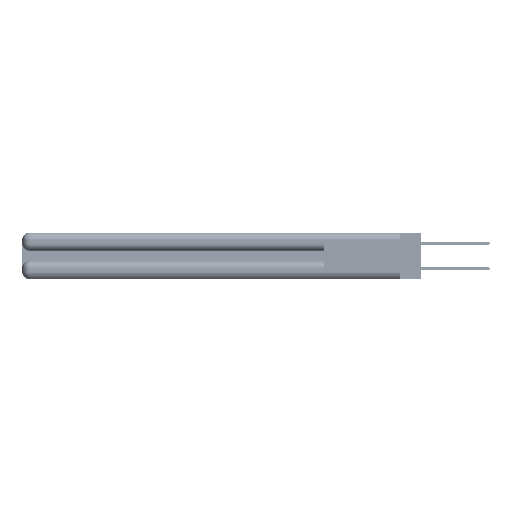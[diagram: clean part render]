
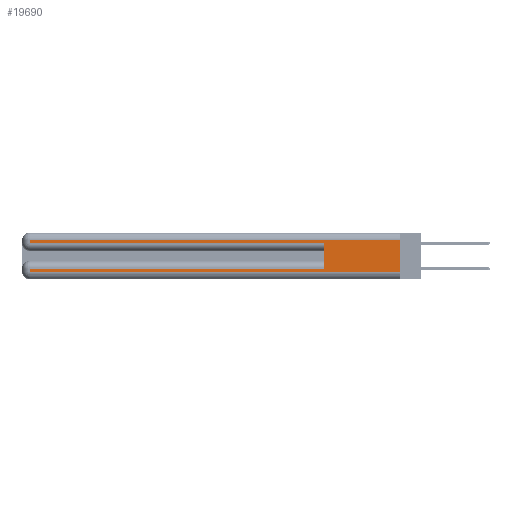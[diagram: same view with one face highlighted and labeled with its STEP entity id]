
A CAD part, left-side view. The second image highlights one B-rep face of the part: STEP entity #19690.
In plain terms, the highlighted planar face has unit normal (-1, 0, 0).
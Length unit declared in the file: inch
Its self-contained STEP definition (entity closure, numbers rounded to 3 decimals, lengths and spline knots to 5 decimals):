
#642 = EDGE_CURVE ( 'NONE', #25531, #5206, #15924, .T. ) ;
#791 = DIRECTION ( 'NONE',  ( 0., 0., -1. ) ) ;
#2185 = LINE ( 'NONE', #38076, #24866 ) ;
#4907 = PLANE ( 'NONE',  #18648 ) ;
#5204 = ORIENTED_EDGE ( 'NONE', *, *, #642, .F. ) ;
#5206 = VERTEX_POINT ( 'NONE', #48222 ) ;
#6239 = VECTOR ( 'NONE', #22172, 39.37008 ) ;
#6719 = VECTOR ( 'NONE', #21812, 39.37008 ) ;
#8620 = CARTESIAN_POINT ( 'NONE',  ( 0., 0., 0.31 ) ) ;
#8904 = EDGE_LOOP ( 'NONE', ( #52292, #32001, #41265, #22554, #5204, #45178, #51805, #26431 ) ) ;
#9344 = LINE ( 'NONE', #25395, #31962 ) ;
#10010 = EDGE_CURVE ( 'NONE', #43387, #15012, #35726, .T. ) ;
#10429 = VECTOR ( 'NONE', #53591, 39.37008 ) ;
#13871 = DIRECTION ( 'NONE',  ( 0., 1., 0. ) ) ;
#14803 = VERTEX_POINT ( 'NONE', #8620 ) ;
#15012 = VERTEX_POINT ( 'NONE', #43968 ) ;
#15924 = LINE ( 'NONE', #39296, #37211 ) ;
#16337 = CARTESIAN_POINT ( 'NONE',  ( 0., 2.94, 0.285 ) ) ;
#17550 = CARTESIAN_POINT ( 'NONE',  ( 0., 2.94, 0.37 ) ) ;
#17668 = EDGE_CURVE ( 'NONE', #43032, #5206, #2185, .T. ) ;
#17908 = CARTESIAN_POINT ( 'NONE',  ( 0., 0., 0.37 ) ) ;
#18648 = AXIS2_PLACEMENT_3D ( 'NONE', #43265, #26305, #791 ) ;
#19479 = CARTESIAN_POINT ( 'NONE',  ( 0., 0., 0.06 ) ) ;
#19516 = EDGE_CURVE ( 'NONE', #14803, #42316, #9344, .T. ) ;
#19690 = ADVANCED_FACE ( 'NONE', ( #33978 ), #4907, .F. ) ;
#21027 = CARTESIAN_POINT ( 'NONE',  ( 0., 2.94, 0.085 ) ) ;
#21812 = DIRECTION ( 'NONE',  ( 0., 0., -1. ) ) ;
#21819 = EDGE_CURVE ( 'NONE', #42316, #43032, #52481, .T. ) ;
#22172 = DIRECTION ( 'NONE',  ( 0., 0., -1. ) ) ;
#22333 = DIRECTION ( 'NONE',  ( 0., 0., 1. ) ) ;
#22554 = ORIENTED_EDGE ( 'NONE', *, *, #17668, .T. ) ;
#23905 = CARTESIAN_POINT ( 'NONE',  ( 0., 0.6, 0.085 ) ) ;
#24866 = VECTOR ( 'NONE', #42327, 39.37008 ) ;
#25395 = CARTESIAN_POINT ( 'NONE',  ( 0., 0., 0.31 ) ) ;
#25531 = VERTEX_POINT ( 'NONE', #23905 ) ;
#26305 = DIRECTION ( 'NONE',  ( 1., 0., 0. ) ) ;
#26395 = VERTEX_POINT ( 'NONE', #21027 ) ;
#26431 = ORIENTED_EDGE ( 'NONE', *, *, #10010, .T. ) ;
#26536 = EDGE_CURVE ( 'NONE', #14803, #15012, #51573, .T. ) ;
#28405 = EDGE_CURVE ( 'NONE', #26395, #43387, #40731, .T. ) ;
#29588 = VECTOR ( 'NONE', #13871, 39.37008 ) ;
#31962 = VECTOR ( 'NONE', #50518, 39.37008 ) ;
#32001 = ORIENTED_EDGE ( 'NONE', *, *, #19516, .T. ) ;
#33978 = FACE_OUTER_BOUND ( 'NONE', #8904, .T. ) ;
#35659 = CARTESIAN_POINT ( 'NONE',  ( 0., 2.94, 0.06 ) ) ;
#35726 = LINE ( 'NONE', #19479, #10429 ) ;
#37211 = VECTOR ( 'NONE', #22333, 39.37008 ) ;
#38076 = CARTESIAN_POINT ( 'NONE',  ( 0., 0., 0.285 ) ) ;
#39296 = CARTESIAN_POINT ( 'NONE',  ( 0., 0.6, 0.145 ) ) ;
#39333 = CARTESIAN_POINT ( 'NONE',  ( 0., 0., 0.085 ) ) ;
#39804 = VECTOR ( 'NONE', #52495, 39.37008 ) ;
#40731 = LINE ( 'NONE', #17550, #6719 ) ;
#41265 = ORIENTED_EDGE ( 'NONE', *, *, #21819, .T. ) ;
#42316 = VERTEX_POINT ( 'NONE', #50301 ) ;
#42327 = DIRECTION ( 'NONE',  ( 0., -1., 0. ) ) ;
#43032 = VERTEX_POINT ( 'NONE', #16337 ) ;
#43265 = CARTESIAN_POINT ( 'NONE',  ( 0., 0., 0.37 ) ) ;
#43387 = VERTEX_POINT ( 'NONE', #35659 ) ;
#43968 = CARTESIAN_POINT ( 'NONE',  ( 0., 0., 0.06 ) ) ;
#43998 = EDGE_CURVE ( 'NONE', #25531, #26395, #52252, .T. ) ;
#45178 = ORIENTED_EDGE ( 'NONE', *, *, #43998, .T. ) ;
#48222 = CARTESIAN_POINT ( 'NONE',  ( 0., 0.6, 0.285 ) ) ;
#50301 = CARTESIAN_POINT ( 'NONE',  ( 0., 2.94, 0.31 ) ) ;
#50518 = DIRECTION ( 'NONE',  ( 0., 1., 0. ) ) ;
#51573 = LINE ( 'NONE', #17908, #6239 ) ;
#51805 = ORIENTED_EDGE ( 'NONE', *, *, #28405, .T. ) ;
#52252 = LINE ( 'NONE', #39333, #29588 ) ;
#52292 = ORIENTED_EDGE ( 'NONE', *, *, #26536, .F. ) ;
#52313 = CARTESIAN_POINT ( 'NONE',  ( 0., 2.94, 0.37 ) ) ;
#52481 = LINE ( 'NONE', #52313, #39804 ) ;
#52495 = DIRECTION ( 'NONE',  ( 0., 0., -1. ) ) ;
#53591 = DIRECTION ( 'NONE',  ( 0., -1., 0. ) ) ;
